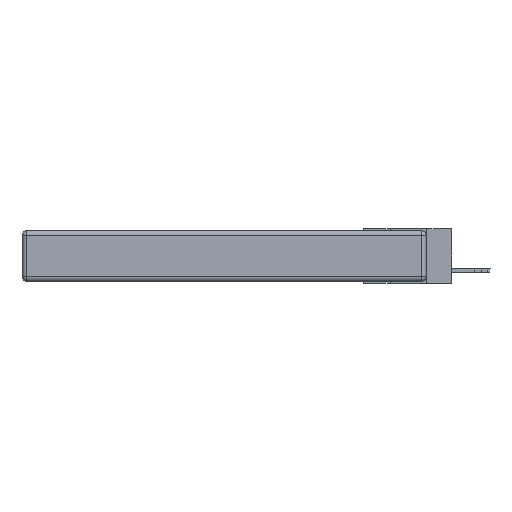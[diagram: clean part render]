
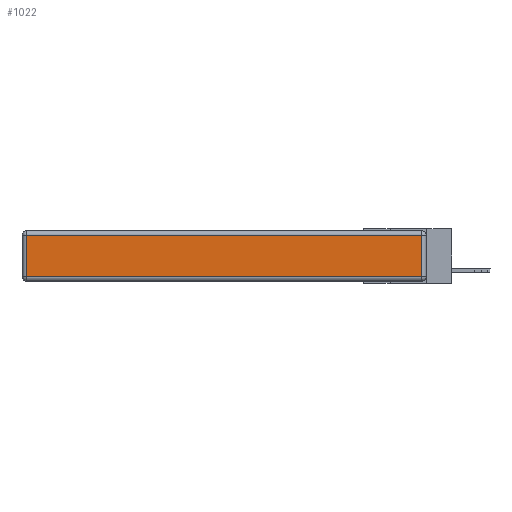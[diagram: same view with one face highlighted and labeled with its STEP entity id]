
A CAD part, left-side view. The second image highlights one B-rep face of the part: STEP entity #1022.
In plain terms, the highlighted planar face has unit normal (-1, 0, 0).
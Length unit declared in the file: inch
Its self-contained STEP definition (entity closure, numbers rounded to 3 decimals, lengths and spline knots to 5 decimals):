
#192 = FACE_OUTER_BOUND ( 'NONE', #3665, .T. ) ;
#433 = VECTOR ( 'NONE', #13717, 39.37008 ) ;
#892 = VERTEX_POINT ( 'NONE', #10766 ) ;
#1005 = AXIS2_PLACEMENT_3D ( 'NONE', #2256, #6536, #2301 ) ;
#1022 = ADVANCED_FACE ( 'NONE', ( #192 ), #9836, .T. ) ;
#1078 = VERTEX_POINT ( 'NONE', #8001 ) ;
#1284 = EDGE_CURVE ( 'NONE', #1078, #892, #5798, .T. ) ;
#1350 = DIRECTION ( 'NONE',  ( 0., 0., 1. ) ) ;
#1584 = VECTOR ( 'NONE', #13311, 39.37008 ) ;
#1754 = LINE ( 'NONE', #4746, #1584 ) ;
#1903 = CARTESIAN_POINT ( 'NONE',  ( 0., 2.75, -0.03 ) ) ;
#2030 = DIRECTION ( 'NONE',  ( 0., 1., 0. ) ) ;
#2138 = CARTESIAN_POINT ( 'NONE',  ( 0., 2.72, -0.313 ) ) ;
#2256 = CARTESIAN_POINT ( 'NONE',  ( 0., 0., -0.343 ) ) ;
#2301 = DIRECTION ( 'NONE',  ( 0., 0., 1. ) ) ;
#2582 = CARTESIAN_POINT ( 'NONE',  ( 0., 0.03, -0.343 ) ) ;
#3187 = EDGE_CURVE ( 'NONE', #9371, #1078, #3747, .T. ) ;
#3446 = ORIENTED_EDGE ( 'NONE', *, *, #3187, .T. ) ;
#3535 = CARTESIAN_POINT ( 'NONE',  ( 0., 0.03, -0.313 ) ) ;
#3665 = EDGE_LOOP ( 'NONE', ( #5521, #3446, #3998, #9245 ) ) ;
#3747 = LINE ( 'NONE', #2582, #4429 ) ;
#3998 = ORIENTED_EDGE ( 'NONE', *, *, #1284, .T. ) ;
#4429 = VECTOR ( 'NONE', #1350, 39.37008 ) ;
#4746 = CARTESIAN_POINT ( 'NONE',  ( 0., 2.72, -0.343 ) ) ;
#5521 = ORIENTED_EDGE ( 'NONE', *, *, #6384, .T. ) ;
#5798 = LINE ( 'NONE', #1903, #10817 ) ;
#6384 = EDGE_CURVE ( 'NONE', #6822, #9371, #7875, .T. ) ;
#6536 = DIRECTION ( 'NONE',  ( -1., 0., 0. ) ) ;
#6822 = VERTEX_POINT ( 'NONE', #2138 ) ;
#7875 = LINE ( 'NONE', #8362, #433 ) ;
#8001 = CARTESIAN_POINT ( 'NONE',  ( 0., 0.03, -0.03 ) ) ;
#8362 = CARTESIAN_POINT ( 'NONE',  ( 0., 0., -0.313 ) ) ;
#9245 = ORIENTED_EDGE ( 'NONE', *, *, #12236, .T. ) ;
#9371 = VERTEX_POINT ( 'NONE', #3535 ) ;
#9836 = PLANE ( 'NONE',  #1005 ) ;
#10766 = CARTESIAN_POINT ( 'NONE',  ( 0., 2.72, -0.03 ) ) ;
#10817 = VECTOR ( 'NONE', #2030, 39.37008 ) ;
#12236 = EDGE_CURVE ( 'NONE', #892, #6822, #1754, .T. ) ;
#13311 = DIRECTION ( 'NONE',  ( 0., 0., -1. ) ) ;
#13717 = DIRECTION ( 'NONE',  ( 0., -1., 0. ) ) ;
